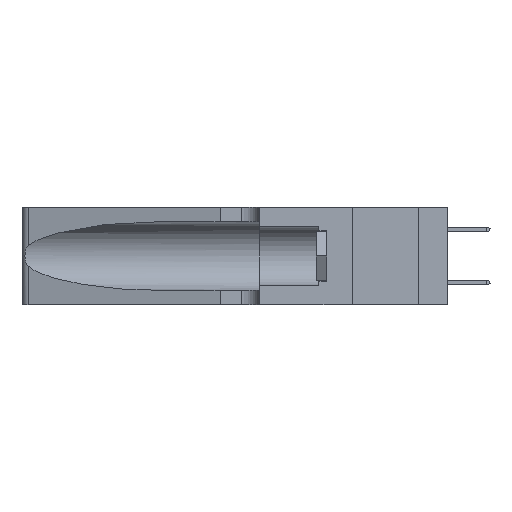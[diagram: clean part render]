
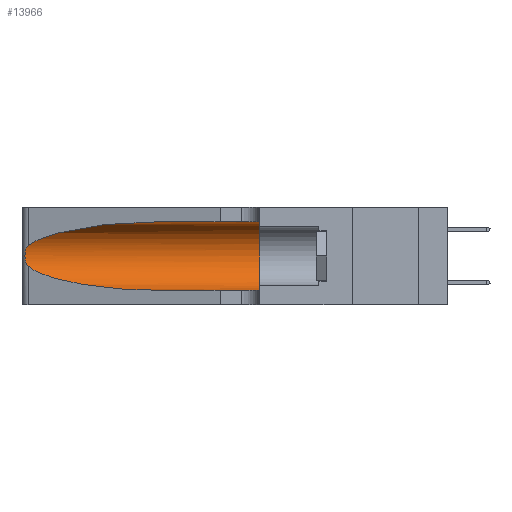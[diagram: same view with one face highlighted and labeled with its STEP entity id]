
A CAD part, left-side view. The second image highlights one B-rep face of the part: STEP entity #13966.
In plain terms, the highlighted cylindrical face has radius 3.308 mm (diameter 6.617 mm), a partial arc.
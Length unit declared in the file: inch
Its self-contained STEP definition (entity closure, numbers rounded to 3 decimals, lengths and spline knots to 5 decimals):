
#386 = CARTESIAN_POINT ( 'NONE',  ( 0.25487, 1.22718, 0.22369 ) ) ;
#629 = EDGE_CURVE ( 'NONE', #39764, #4839, #39498, .T. ) ;
#1221 = DIRECTION ( 'NONE',  ( 0., 1., 0. ) ) ;
#1484 = EDGE_CURVE ( 'NONE', #4703, #16210, #42561, .T. ) ;
#2279 = CYLINDRICAL_SURFACE ( 'NONE', #38730, 0.13025 ) ;
#2398 = CARTESIAN_POINT ( 'NONE',  ( 0.26018, 1.23835, 0.19895 ) ) ;
#2670 = CARTESIAN_POINT ( 'NONE',  ( 0.25487, 1.22718, 0.22369 ) ) ;
#2683 = CARTESIAN_POINT ( 'NONE',  ( 0.25555, 1.22994, 0.2215 ) ) ;
#3414 = ORIENTED_EDGE ( 'NONE', *, *, #39580, .T. ) ;
#3826 = CARTESIAN_POINT ( 'NONE',  ( 0.1305, 0.72297, 0.05475 ) ) ;
#3930 = CARTESIAN_POINT ( 'NONE',  ( 0.1305, 0.35, 0.05475 ) ) ;
#3976 = CARTESIAN_POINT ( 'NONE',  ( 0.2373, 1.15595, 0.28018 ) ) ;
#4368 = ORIENTED_EDGE ( 'NONE', *, *, #19000, .T. ) ;
#4555 = DIRECTION ( 'NONE',  ( 0., 0., 1. ) ) ;
#4703 = VERTEX_POINT ( 'NONE', #3826 ) ;
#4732 = CARTESIAN_POINT ( 'NONE',  ( 0.25487, 1.22718, 0.14631 ) ) ;
#4839 = VERTEX_POINT ( 'NONE', #20852 ) ;
#5732 = CARTESIAN_POINT ( 'NONE',  ( 0.26017, 1.23833, 0.17102 ) ) ;
#7057 = VECTOR ( 'NONE', #26814, 39.37008 ) ;
#7473 = CARTESIAN_POINT ( 'NONE',  ( 0.1305, 0.35, 0.185 ) ) ;
#12834 = CARTESIAN_POINT ( 'NONE',  ( 0.25555, 1.22993, 0.14849 ) ) ;
#13966 = ADVANCED_FACE ( 'NONE', ( #33540 ), #2279, .F. ) ;
#14710 = AXIS2_PLACEMENT_3D ( 'NONE', #7473, #1221, #4555 ) ;
#15739 = CARTESIAN_POINT ( 'NONE',  ( 0.25856, 1.23593, 0.16098 ) ) ;
#15763 = CARTESIAN_POINT ( 'NONE',  ( 0.25487, 1.22718, 0.14631 ) ) ;
#16034 = CARTESIAN_POINT ( 'NONE',  ( 0.25639, 1.23186, 0.15144 ) ) ;
#16210 = VERTEX_POINT ( 'NONE', #3930 ) ;
#17839 = EDGE_CURVE ( 'NONE', #32309, #30828, #18345, .T. ) ;
#18345 = B_SPLINE_CURVE_WITH_KNOTS ( 'NONE', 3,
 ( #22462, #2683, #35765, #25953, #28899, #2398, #25807, #42200, #5732, #15739, #32691, #16034, #12834, #22743 ),
 .UNSPECIFIED., .F., .F.,
 ( 4, 2, 2, 2, 2, 2, 4 ),
 ( 0., 0.00027, 0.00053, 0.00107, 0.0016, 0.00187, 0.00214 ),
 .UNSPECIFIED. ) ;
#18851 = DIRECTION ( 'NONE',  ( 0., -1., 0. ) ) ;
#18885 =( BOUNDED_CURVE ( )  B_SPLINE_CURVE ( 3, ( #34156, #30789, #3976, #386 ),
 .UNSPECIFIED., .F., .F. ) 
 B_SPLINE_CURVE_WITH_KNOTS ( ( 4, 4 ),
 ( 1.5708, 2.84003 ),
 .UNSPECIFIED. ) 
 CURVE ( )  GEOMETRIC_REPRESENTATION_ITEM ( )  RATIONAL_B_SPLINE_CURVE ( ( 1., 0.87, 0.87, 1. ) ) 
 REPRESENTATION_ITEM ( '' )  );
#19000 = EDGE_CURVE ( 'NONE', #39764, #32309, #18885, .T. ) ;
#20010 = DIRECTION ( 'NONE',  ( 0., -1., 0. ) ) ;
#20454 =( BOUNDED_CURVE ( )  B_SPLINE_CURVE ( 3, ( #15763, #32566, #22345, #40167 ),
 .UNSPECIFIED., .F., .F. ) 
 B_SPLINE_CURVE_WITH_KNOTS ( ( 4, 4 ),
 ( 3.44316, 4.71239 ),
 .UNSPECIFIED. ) 
 CURVE ( )  GEOMETRIC_REPRESENTATION_ITEM ( )  RATIONAL_B_SPLINE_CURVE ( ( 1., 0.87, 0.87, 1. ) ) 
 REPRESENTATION_ITEM ( '' )  );
#20852 = CARTESIAN_POINT ( 'NONE',  ( 0.1305, 0.35, 0.31525 ) ) ;
#21795 = EDGE_LOOP ( 'NONE', ( #4368, #32645, #3414, #22639, #22238, #34167 ) ) ;
#22238 = ORIENTED_EDGE ( 'NONE', *, *, #34668, .F. ) ;
#22345 = CARTESIAN_POINT ( 'NONE',  ( 0.18966, 0.96281, 0.05475 ) ) ;
#22462 = CARTESIAN_POINT ( 'NONE',  ( 0.25487, 1.22718, 0.22369 ) ) ;
#22639 = ORIENTED_EDGE ( 'NONE', *, *, #1484, .T. ) ;
#22743 = CARTESIAN_POINT ( 'NONE',  ( 0.25487, 1.22718, 0.14631 ) ) ;
#23344 = DIRECTION ( 'NONE',  ( 0., 0., -1. ) ) ;
#25807 = CARTESIAN_POINT ( 'NONE',  ( 0.26075, 1.23896, 0.19203 ) ) ;
#25953 = CARTESIAN_POINT ( 'NONE',  ( 0.25787, 1.23484, 0.2124 ) ) ;
#26814 = DIRECTION ( 'NONE',  ( 0., -1., 0. ) ) ;
#28899 = CARTESIAN_POINT ( 'NONE',  ( 0.25854, 1.2359, 0.20912 ) ) ;
#29628 = CARTESIAN_POINT ( 'NONE',  ( 0.1305, 0.72297, 0.31525 ) ) ;
#30467 = CARTESIAN_POINT ( 'NONE',  ( 0.1305, 1.61858, 0.05475 ) ) ;
#30789 = CARTESIAN_POINT ( 'NONE',  ( 0.18966, 0.96281, 0.31525 ) ) ;
#30828 = VERTEX_POINT ( 'NONE', #4732 ) ;
#32309 = VERTEX_POINT ( 'NONE', #2670 ) ;
#32566 = CARTESIAN_POINT ( 'NONE',  ( 0.2373, 1.15595, 0.08982 ) ) ;
#32645 = ORIENTED_EDGE ( 'NONE', *, *, #17839, .T. ) ;
#32691 = CARTESIAN_POINT ( 'NONE',  ( 0.25789, 1.23486, 0.15765 ) ) ;
#33217 = VECTOR ( 'NONE', #18851, 39.37008 ) ;
#33304 = CARTESIAN_POINT ( 'NONE',  ( 0.1305, 1.61858, 0.185 ) ) ;
#33540 = FACE_OUTER_BOUND ( 'NONE', #21795, .T. ) ;
#34156 = CARTESIAN_POINT ( 'NONE',  ( 0.1305, 0.72297, 0.31525 ) ) ;
#34167 = ORIENTED_EDGE ( 'NONE', *, *, #629, .F. ) ;
#34668 = EDGE_CURVE ( 'NONE', #4839, #16210, #42689, .T. ) ;
#35765 = CARTESIAN_POINT ( 'NONE',  ( 0.25639, 1.23184, 0.21858 ) ) ;
#35795 = CARTESIAN_POINT ( 'NONE',  ( 0.1305, 1.61858, 0.31525 ) ) ;
#38730 = AXIS2_PLACEMENT_3D ( 'NONE', #33304, #20010, #23344 ) ;
#39498 = LINE ( 'NONE', #35795, #33217 ) ;
#39580 = EDGE_CURVE ( 'NONE', #30828, #4703, #20454, .T. ) ;
#39764 = VERTEX_POINT ( 'NONE', #29628 ) ;
#40167 = CARTESIAN_POINT ( 'NONE',  ( 0.1305, 0.72297, 0.05475 ) ) ;
#42200 = CARTESIAN_POINT ( 'NONE',  ( 0.26075, 1.23896, 0.178 ) ) ;
#42561 = LINE ( 'NONE', #30467, #7057 ) ;
#42689 = CIRCLE ( 'NONE', #14710, 0.13025 ) ;
